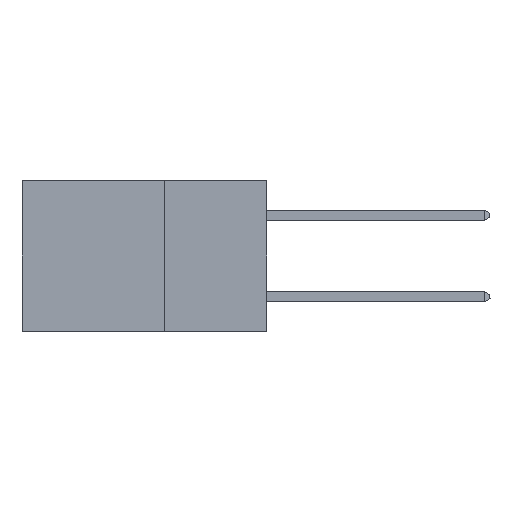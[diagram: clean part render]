
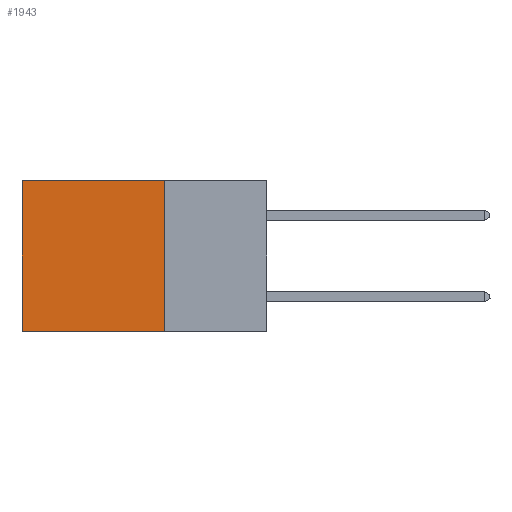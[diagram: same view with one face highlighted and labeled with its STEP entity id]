
A CAD part, left-side view. The second image highlights one B-rep face of the part: STEP entity #1943.
In plain terms, the highlighted planar face has unit normal (-1, 0, 0).
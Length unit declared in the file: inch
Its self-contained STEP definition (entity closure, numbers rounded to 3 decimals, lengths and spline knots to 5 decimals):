
#456 = FACE_OUTER_BOUND ( 'NONE', #32233, .T. ) ;
#1042 = CARTESIAN_POINT ( 'NONE',  ( 0.2875, 0.6, 0. ) ) ;
#1189 = EDGE_CURVE ( 'NONE', #14825, #4661, #31745, .T. ) ;
#1943 = ADVANCED_FACE ( 'NONE', ( #456 ), #12533, .F. ) ;
#1990 = EDGE_CURVE ( 'NONE', #4661, #25368, #26045, .T. ) ;
#4264 = CARTESIAN_POINT ( 'NONE',  ( 0.2875, 0.25, -0.37 ) ) ;
#4661 = VERTEX_POINT ( 'NONE', #21750 ) ;
#5107 = LINE ( 'NONE', #15059, #27088 ) ;
#6071 = EDGE_CURVE ( 'NONE', #22268, #25368, #5107, .T. ) ;
#6904 = AXIS2_PLACEMENT_3D ( 'NONE', #28644, #28839, #16334 ) ;
#7085 = CARTESIAN_POINT ( 'NONE',  ( 0.2875, 0.25, 0. ) ) ;
#8159 = VECTOR ( 'NONE', #10902, 39.37008 ) ;
#9543 = VECTOR ( 'NONE', #31379, 39.37008 ) ;
#10902 = DIRECTION ( 'NONE',  ( 0., 0., -1. ) ) ;
#12533 = PLANE ( 'NONE',  #6904 ) ;
#13808 = CARTESIAN_POINT ( 'NONE',  ( 0.2875, 0.25, 0. ) ) ;
#14825 = VERTEX_POINT ( 'NONE', #37923 ) ;
#15059 = CARTESIAN_POINT ( 'NONE',  ( 0.2875, 0.25, -0.37 ) ) ;
#16122 = VECTOR ( 'NONE', #29320, 39.37008 ) ;
#16334 = DIRECTION ( 'NONE',  ( 0., 0., -1. ) ) ;
#21750 = CARTESIAN_POINT ( 'NONE',  ( 0.2875, 0.6, 0. ) ) ;
#22268 = VERTEX_POINT ( 'NONE', #4264 ) ;
#23140 = CARTESIAN_POINT ( 'NONE',  ( 0.2875, 0.6, -0.37 ) ) ;
#25368 = VERTEX_POINT ( 'NONE', #23140 ) ;
#26045 = LINE ( 'NONE', #1042, #8159 ) ;
#27088 = VECTOR ( 'NONE', #30168, 39.37008 ) ;
#27712 = ORIENTED_EDGE ( 'NONE', *, *, #1189, .T. ) ;
#28644 = CARTESIAN_POINT ( 'NONE',  ( 0.2875, 0.25, 0. ) ) ;
#28839 = DIRECTION ( 'NONE',  ( 1., 0., 0. ) ) ;
#29320 = DIRECTION ( 'NONE',  ( 0., 1., 0. ) ) ;
#30168 = DIRECTION ( 'NONE',  ( 0., 1., 0. ) ) ;
#31379 = DIRECTION ( 'NONE',  ( 0., 0., -1. ) ) ;
#31745 = LINE ( 'NONE', #13808, #16122 ) ;
#32233 = EDGE_LOOP ( 'NONE', ( #34045, #34074, #38292, #27712 ) ) ;
#34045 = ORIENTED_EDGE ( 'NONE', *, *, #1990, .T. ) ;
#34074 = ORIENTED_EDGE ( 'NONE', *, *, #6071, .F. ) ;
#34371 = LINE ( 'NONE', #7085, #9543 ) ;
#36593 = EDGE_CURVE ( 'NONE', #14825, #22268, #34371, .T. ) ;
#37923 = CARTESIAN_POINT ( 'NONE',  ( 0.2875, 0.25, 0. ) ) ;
#38292 = ORIENTED_EDGE ( 'NONE', *, *, #36593, .F. ) ;
